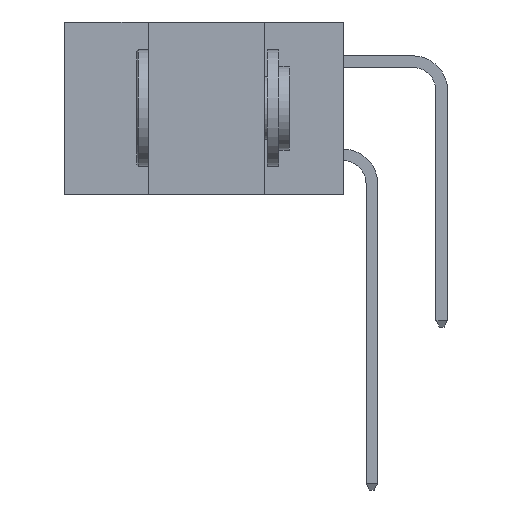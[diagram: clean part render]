
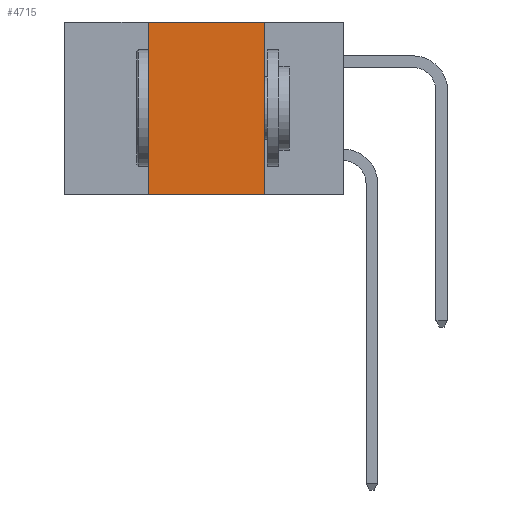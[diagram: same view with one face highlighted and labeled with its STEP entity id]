
A CAD part, left-side view. The second image highlights one B-rep face of the part: STEP entity #4715.
In plain terms, the highlighted planar face has unit normal (-1, 0, 0).
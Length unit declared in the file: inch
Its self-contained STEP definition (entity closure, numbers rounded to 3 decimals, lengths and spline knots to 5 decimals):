
#36 = ORIENTED_EDGE ( 'NONE', *, *, #12683, .F. ) ;
#146 = LINE ( 'NONE', #3723, #14601 ) ;
#2445 = ORIENTED_EDGE ( 'NONE', *, *, #19966, .T. ) ;
#2951 = LINE ( 'NONE', #22203, #8029 ) ;
#3039 = VECTOR ( 'NONE', #11186, 39.37008 ) ;
#3723 = CARTESIAN_POINT ( 'NONE',  ( 0., 0.17, -0.37 ) ) ;
#4715 = ADVANCED_FACE ( 'NONE', ( #10049 ), #5440, .F. ) ;
#5384 = DIRECTION ( 'NONE',  ( 0., 0., -1. ) ) ;
#5433 = DIRECTION ( 'NONE',  ( 1., 0., 0. ) ) ;
#5440 = PLANE ( 'NONE',  #15396 ) ;
#5969 = CARTESIAN_POINT ( 'NONE',  ( 0., 0.6, 0. ) ) ;
#7105 = VERTEX_POINT ( 'NONE', #14941 ) ;
#7567 = DIRECTION ( 'NONE',  ( 0., -1., 0. ) ) ;
#8029 = VECTOR ( 'NONE', #7567, 39.37008 ) ;
#8168 = VECTOR ( 'NONE', #22085, 39.37008 ) ;
#8713 = LINE ( 'NONE', #22072, #3039 ) ;
#9607 = CARTESIAN_POINT ( 'NONE',  ( 0., 0.17, -0.37 ) ) ;
#10049 = FACE_OUTER_BOUND ( 'NONE', #11342, .T. ) ;
#11186 = DIRECTION ( 'NONE',  ( 0., 0., 1. ) ) ;
#11200 = CARTESIAN_POINT ( 'NONE',  ( 0., 0.6, 0. ) ) ;
#11342 = EDGE_LOOP ( 'NONE', ( #36, #12804, #16724, #2445 ) ) ;
#12466 = VERTEX_POINT ( 'NONE', #23362 ) ;
#12683 = EDGE_CURVE ( 'NONE', #7105, #22367, #146, .T. ) ;
#12804 = ORIENTED_EDGE ( 'NONE', *, *, #13906, .F. ) ;
#13375 = VERTEX_POINT ( 'NONE', #22493 ) ;
#13906 = EDGE_CURVE ( 'NONE', #12466, #7105, #22709, .T. ) ;
#14601 = VECTOR ( 'NONE', #18621, 39.37008 ) ;
#14941 = CARTESIAN_POINT ( 'NONE',  ( 0., 0.17, 0. ) ) ;
#15396 = AXIS2_PLACEMENT_3D ( 'NONE', #5969, #5433, #5384 ) ;
#16724 = ORIENTED_EDGE ( 'NONE', *, *, #17583, .F. ) ;
#17583 = EDGE_CURVE ( 'NONE', #13375, #12466, #8713, .T. ) ;
#18621 = DIRECTION ( 'NONE',  ( 0., 0., -1. ) ) ;
#19966 = EDGE_CURVE ( 'NONE', #13375, #22367, #2951, .T. ) ;
#22072 = CARTESIAN_POINT ( 'NONE',  ( 0., 0.42, -0.37 ) ) ;
#22085 = DIRECTION ( 'NONE',  ( 0., -1., 0. ) ) ;
#22203 = CARTESIAN_POINT ( 'NONE',  ( 0., 0.6, -0.37 ) ) ;
#22367 = VERTEX_POINT ( 'NONE', #9607 ) ;
#22493 = CARTESIAN_POINT ( 'NONE',  ( 0., 0.42, -0.37 ) ) ;
#22709 = LINE ( 'NONE', #11200, #8168 ) ;
#23362 = CARTESIAN_POINT ( 'NONE',  ( 0., 0.42, 0. ) ) ;
